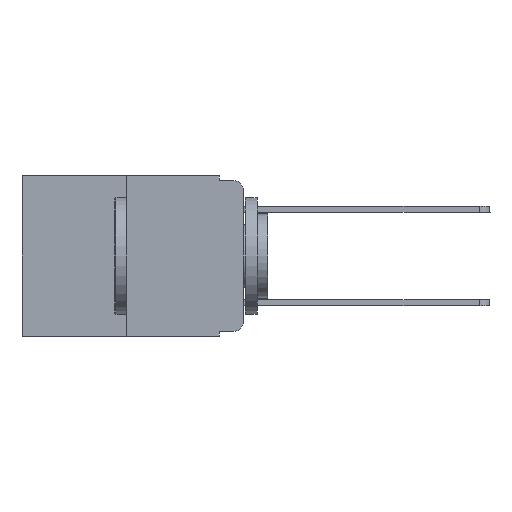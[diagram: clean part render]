
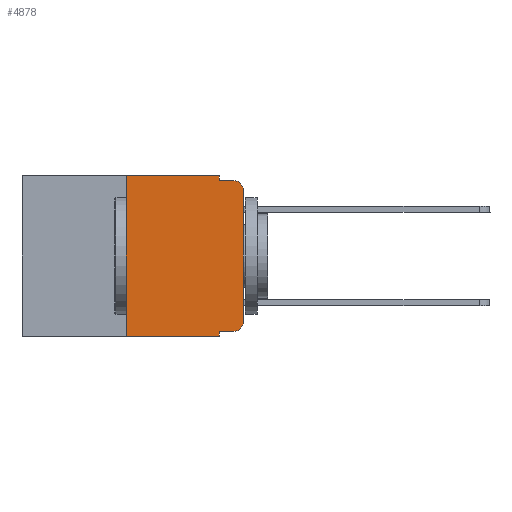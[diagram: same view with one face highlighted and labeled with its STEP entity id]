
A CAD part, left-side view. The second image highlights one B-rep face of the part: STEP entity #4878.
In plain terms, the highlighted planar face has unit normal (-1, 0, 0).
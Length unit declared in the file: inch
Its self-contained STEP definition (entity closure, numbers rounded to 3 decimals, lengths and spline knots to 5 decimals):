
#218 = VERTEX_POINT ( 'NONE', #7624 ) ;
#745 = CARTESIAN_POINT ( 'NONE',  ( 0., 0.051, 0. ) ) ;
#1218 = FACE_OUTER_BOUND ( 'NONE', #8750, .T. ) ;
#1375 = VECTOR ( 'NONE', #12458, 39.37008 ) ;
#1479 = DIRECTION ( 'NONE',  ( 0., -1., 0. ) ) ;
#1677 = DIRECTION ( 'NONE',  ( 0., -1., 0. ) ) ;
#1693 = CARTESIAN_POINT ( 'NONE',  ( 0., 0.02, -0.313 ) ) ;
#1793 = CARTESIAN_POINT ( 'NONE',  ( 0., 0.473, 0. ) ) ;
#1921 = DIRECTION ( 'NONE',  ( 0., -1., 0. ) ) ;
#2300 = EDGE_CURVE ( 'NONE', #17337, #9878, #4966, .T. ) ;
#2770 = EDGE_CURVE ( 'NONE', #18464, #23399, #9553, .T. ) ;
#2798 = LINE ( 'NONE', #20063, #8311 ) ;
#3783 = DIRECTION ( 'NONE',  ( 0., -1., 0. ) ) ;
#3803 = ORIENTED_EDGE ( 'NONE', *, *, #10041, .T. ) ;
#3816 = VECTOR ( 'NONE', #7033, 39.37008 ) ;
#4348 = DIRECTION ( 'NONE',  ( -1., 0., 0. ) ) ;
#4575 = LINE ( 'NONE', #23487, #15532 ) ;
#4817 = LINE ( 'NONE', #5406, #10896 ) ;
#4878 = ADVANCED_FACE ( 'NONE', ( #1218 ), #18045, .F. ) ;
#4966 = LINE ( 'NONE', #5214, #19068 ) ;
#5214 = CARTESIAN_POINT ( 'NONE',  ( 0., 0.051, -0.01 ) ) ;
#5241 = DIRECTION ( 'NONE',  ( 0., 0., -1. ) ) ;
#5251 = VERTEX_POINT ( 'NONE', #745 ) ;
#5313 = CARTESIAN_POINT ( 'NONE',  ( 0., 0., -0.03 ) ) ;
#5398 = DIRECTION ( 'NONE',  ( -1., 0., 0. ) ) ;
#5406 = CARTESIAN_POINT ( 'NONE',  ( 0., 0.473, 0. ) ) ;
#5414 = LINE ( 'NONE', #12309, #1375 ) ;
#5552 = EDGE_CURVE ( 'NONE', #9514, #12306, #10723, .T. ) ;
#5687 = LINE ( 'NONE', #14446, #15792 ) ;
#5933 = ORIENTED_EDGE ( 'NONE', *, *, #2300, .F. ) ;
#6683 = CARTESIAN_POINT ( 'NONE',  ( 0., 0.25, 0. ) ) ;
#7033 = DIRECTION ( 'NONE',  ( 0., 0., -1. ) ) ;
#7624 = CARTESIAN_POINT ( 'NONE',  ( 0., 0.051, -0.343 ) ) ;
#7815 = VECTOR ( 'NONE', #13055, 39.37008 ) ;
#8311 = VECTOR ( 'NONE', #1921, 39.37008 ) ;
#8750 = EDGE_LOOP ( 'NONE', ( #19260, #13166, #5933, #17974, #22332, #18093, #18358, #17581, #3803, #23320 ) ) ;
#9165 = DIRECTION ( 'NONE',  ( 1., 0., 0. ) ) ;
#9207 = CARTESIAN_POINT ( 'NONE',  ( 0., 0.25, 0. ) ) ;
#9514 = VERTEX_POINT ( 'NONE', #16835 ) ;
#9553 = LINE ( 'NONE', #6683, #7815 ) ;
#9783 = EDGE_CURVE ( 'NONE', #12306, #23417, #5414, .T. ) ;
#9824 = EDGE_CURVE ( 'NONE', #5251, #17337, #5687, .T. ) ;
#9878 = VERTEX_POINT ( 'NONE', #21736 ) ;
#9932 = EDGE_CURVE ( 'NONE', #23399, #5251, #4817, .T. ) ;
#10041 = EDGE_CURVE ( 'NONE', #11575, #9514, #2798, .T. ) ;
#10723 = CIRCLE ( 'NONE', #23134, 0.02 ) ;
#10896 = VECTOR ( 'NONE', #3783, 39.37008 ) ;
#11575 = VERTEX_POINT ( 'NONE', #18962 ) ;
#12306 = VERTEX_POINT ( 'NONE', #19196 ) ;
#12309 = CARTESIAN_POINT ( 'NONE',  ( 0., 0., 0. ) ) ;
#12458 = DIRECTION ( 'NONE',  ( 0., 0., 1. ) ) ;
#12511 = EDGE_CURVE ( 'NONE', #11575, #218, #21391, .T. ) ;
#12623 = CARTESIAN_POINT ( 'NONE',  ( 0., 0.051, 0. ) ) ;
#12815 = AXIS2_PLACEMENT_3D ( 'NONE', #1793, #9165, #13064 ) ;
#13055 = DIRECTION ( 'NONE',  ( 0., 0., 1. ) ) ;
#13064 = DIRECTION ( 'NONE',  ( 0., 0., -1. ) ) ;
#13166 = ORIENTED_EDGE ( 'NONE', *, *, #14822, .T. ) ;
#13268 = AXIS2_PLACEMENT_3D ( 'NONE', #21081, #4348, #22968 ) ;
#13326 = DIRECTION ( 'NONE',  ( 0., 0., -1. ) ) ;
#14388 = CIRCLE ( 'NONE', #13268, 0.02 ) ;
#14446 = CARTESIAN_POINT ( 'NONE',  ( 0., 0.051, 0. ) ) ;
#14822 = EDGE_CURVE ( 'NONE', #23417, #9878, #14388, .T. ) ;
#15532 = VECTOR ( 'NONE', #1479, 39.37008 ) ;
#15792 = VECTOR ( 'NONE', #5241, 39.37008 ) ;
#16158 = CARTESIAN_POINT ( 'NONE',  ( 0., 0.25, -0.343 ) ) ;
#16835 = CARTESIAN_POINT ( 'NONE',  ( 0., 0.02, -0.333 ) ) ;
#16847 = CARTESIAN_POINT ( 'NONE',  ( 0., 0.051, -0.01 ) ) ;
#17337 = VERTEX_POINT ( 'NONE', #16847 ) ;
#17581 = ORIENTED_EDGE ( 'NONE', *, *, #12511, .F. ) ;
#17974 = ORIENTED_EDGE ( 'NONE', *, *, #9824, .F. ) ;
#18045 = PLANE ( 'NONE',  #12815 ) ;
#18093 = ORIENTED_EDGE ( 'NONE', *, *, #2770, .F. ) ;
#18358 = ORIENTED_EDGE ( 'NONE', *, *, #19141, .T. ) ;
#18464 = VERTEX_POINT ( 'NONE', #16158 ) ;
#18962 = CARTESIAN_POINT ( 'NONE',  ( 0., 0.051, -0.333 ) ) ;
#19068 = VECTOR ( 'NONE', #1677, 39.37008 ) ;
#19141 = EDGE_CURVE ( 'NONE', #18464, #218, #4575, .T. ) ;
#19196 = CARTESIAN_POINT ( 'NONE',  ( 0., 0., -0.313 ) ) ;
#19260 = ORIENTED_EDGE ( 'NONE', *, *, #9783, .T. ) ;
#20063 = CARTESIAN_POINT ( 'NONE',  ( 0., 0.051, -0.333 ) ) ;
#21081 = CARTESIAN_POINT ( 'NONE',  ( 0., 0.02, -0.03 ) ) ;
#21391 = LINE ( 'NONE', #12623, #3816 ) ;
#21736 = CARTESIAN_POINT ( 'NONE',  ( 0., 0.02, -0.01 ) ) ;
#22332 = ORIENTED_EDGE ( 'NONE', *, *, #9932, .F. ) ;
#22968 = DIRECTION ( 'NONE',  ( 0., 0., -1. ) ) ;
#23134 = AXIS2_PLACEMENT_3D ( 'NONE', #1693, #5398, #13326 ) ;
#23320 = ORIENTED_EDGE ( 'NONE', *, *, #5552, .T. ) ;
#23399 = VERTEX_POINT ( 'NONE', #9207 ) ;
#23417 = VERTEX_POINT ( 'NONE', #5313 ) ;
#23487 = CARTESIAN_POINT ( 'NONE',  ( 0., 0.473, -0.343 ) ) ;
